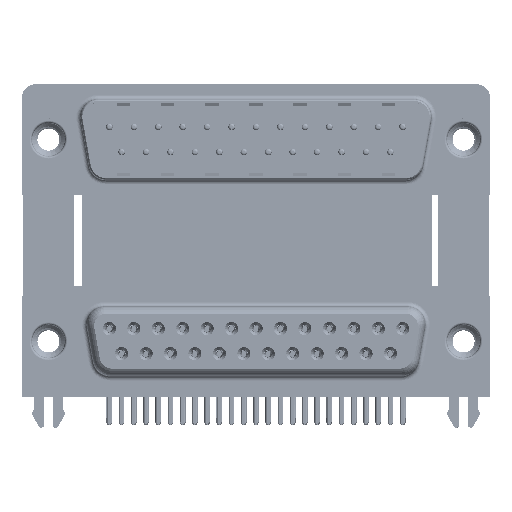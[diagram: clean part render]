
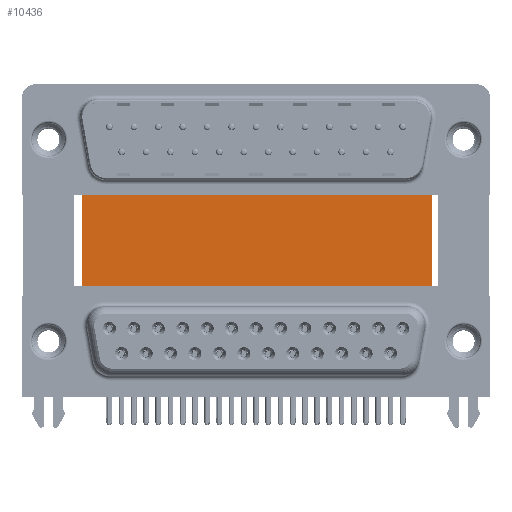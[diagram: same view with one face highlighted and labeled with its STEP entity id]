
A CAD part, top view. The second image highlights one B-rep face of the part: STEP entity #10436.
In plain terms, the highlighted planar face has unit normal (0, 0, 1).
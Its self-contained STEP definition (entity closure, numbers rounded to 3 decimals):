
#2403 = EDGE_CURVE ( 'NONE', #33314, #38773, #8173, .T. ) ;
#5675 = DIRECTION ( 'NONE',  ( 1., 0., 0. ) ) ;
#6084 = DIRECTION ( 'NONE',  ( 0., -1., 0. ) ) ;
#6503 = CARTESIAN_POINT ( 'NONE',  ( 43.43, -3.735, -12. ) ) ;
#6765 = ORIENTED_EDGE ( 'NONE', *, *, #31185, .F. ) ;
#8173 = LINE ( 'NONE', #52666, #31479 ) ;
#8244 = DIRECTION ( 'NONE',  ( 0., 0., -1. ) ) ;
#10436 = ADVANCED_FACE ( 'NONE', ( #21370 ), #34712, .F. ) ;
#11043 = CARTESIAN_POINT ( 'NONE',  ( 3.79, 16.585, -12. ) ) ;
#11203 = CARTESIAN_POINT ( 'NONE',  ( 3.79, -3.735, -12. ) ) ;
#12097 = EDGE_LOOP ( 'NONE', ( #16125, #6765, #23573, #46476 ) ) ;
#16125 = ORIENTED_EDGE ( 'NONE', *, *, #48456, .T. ) ;
#16346 = DIRECTION ( 'NONE',  ( 1., 0., 0. ) ) ;
#18349 = DIRECTION ( 'NONE',  ( 0., -1., 0. ) ) ;
#19209 = LINE ( 'NONE', #11043, #44507 ) ;
#21370 = FACE_OUTER_BOUND ( 'NONE', #12097, .T. ) ;
#23573 = ORIENTED_EDGE ( 'NONE', *, *, #2403, .F. ) ;
#23845 = VECTOR ( 'NONE', #18349, 1000. ) ;
#26015 = DIRECTION ( 'NONE',  ( -1., 0., 0. ) ) ;
#31185 = EDGE_CURVE ( 'NONE', #38773, #40651, #48295, .T. ) ;
#31479 = VECTOR ( 'NONE', #16346, 1000. ) ;
#33314 = VERTEX_POINT ( 'NONE', #40584 ) ;
#34712 = PLANE ( 'NONE',  #38642 ) ;
#38642 = AXIS2_PLACEMENT_3D ( 'NONE', #43411, #8244, #26015 ) ;
#38773 = VERTEX_POINT ( 'NONE', #50833 ) ;
#40584 = CARTESIAN_POINT ( 'NONE',  ( 3.79, 16.585, -12. ) ) ;
#40651 = VERTEX_POINT ( 'NONE', #6503 ) ;
#41990 = VECTOR ( 'NONE', #5675, 1000. ) ;
#43411 = CARTESIAN_POINT ( 'NONE',  ( 3.79, 16.585, -12. ) ) ;
#44446 = EDGE_CURVE ( 'NONE', #33314, #49728, #19209, .T. ) ;
#44502 = CARTESIAN_POINT ( 'NONE',  ( 43.43, 16.585, -12. ) ) ;
#44507 = VECTOR ( 'NONE', #6084, 1000. ) ;
#46476 = ORIENTED_EDGE ( 'NONE', *, *, #44446, .T. ) ;
#48295 = LINE ( 'NONE', #44502, #23845 ) ;
#48456 = EDGE_CURVE ( 'NONE', #49728, #40651, #51033, .T. ) ;
#49728 = VERTEX_POINT ( 'NONE', #51043 ) ;
#50833 = CARTESIAN_POINT ( 'NONE',  ( 43.43, 16.585, -12. ) ) ;
#51033 = LINE ( 'NONE', #11203, #41990 ) ;
#51043 = CARTESIAN_POINT ( 'NONE',  ( 3.79, -3.735, -12. ) ) ;
#52666 = CARTESIAN_POINT ( 'NONE',  ( 3.79, 16.585, -12. ) ) ;
